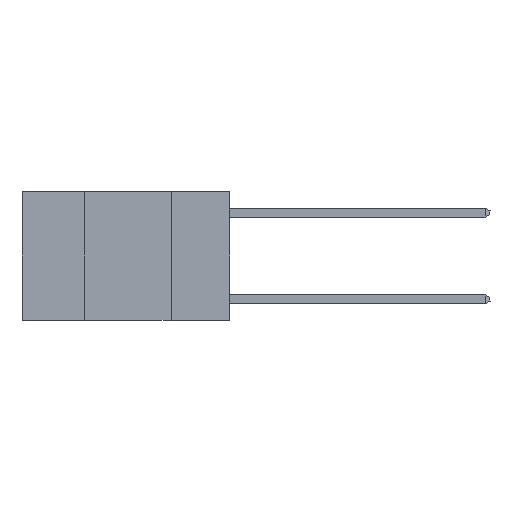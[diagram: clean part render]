
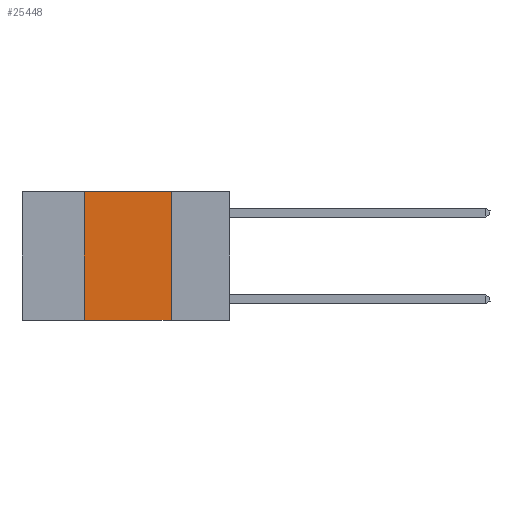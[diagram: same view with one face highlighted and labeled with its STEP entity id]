
A CAD part, left-side view. The second image highlights one B-rep face of the part: STEP entity #25448.
In plain terms, the highlighted planar face has unit normal (-1, 0, 0).
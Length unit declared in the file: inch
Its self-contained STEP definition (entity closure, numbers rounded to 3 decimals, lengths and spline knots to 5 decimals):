
#2127 = FACE_OUTER_BOUND ( 'NONE', #8134, .T. ) ;
#3153 = LINE ( 'NONE', #24647, #7280 ) ;
#5910 = EDGE_CURVE ( 'NONE', #15060, #19365, #3153, .T. ) ;
#6557 = VERTEX_POINT ( 'NONE', #20426 ) ;
#6738 = ORIENTED_EDGE ( 'NONE', *, *, #5910, .F. ) ;
#7203 = CARTESIAN_POINT ( 'NONE',  ( 0., 0.17, -0.37 ) ) ;
#7280 = VECTOR ( 'NONE', #15128, 39.37008 ) ;
#7332 = CARTESIAN_POINT ( 'NONE',  ( 0., 0.42, 0. ) ) ;
#8134 = EDGE_LOOP ( 'NONE', ( #16876, #6738, #12504, #13567 ) ) ;
#9075 = LINE ( 'NONE', #18094, #24394 ) ;
#9433 = EDGE_CURVE ( 'NONE', #6557, #15060, #9075, .T. ) ;
#12504 = ORIENTED_EDGE ( 'NONE', *, *, #9433, .F. ) ;
#13567 = ORIENTED_EDGE ( 'NONE', *, *, #25311, .T. ) ;
#13873 = CARTESIAN_POINT ( 'NONE',  ( 0., 0.6, -0.37 ) ) ;
#15060 = VERTEX_POINT ( 'NONE', #7332 ) ;
#15128 = DIRECTION ( 'NONE',  ( 0., -1., 0. ) ) ;
#15436 = CARTESIAN_POINT ( 'NONE',  ( 0., 0.6, 0. ) ) ;
#15563 = AXIS2_PLACEMENT_3D ( 'NONE', #15436, #29127, #24513 ) ;
#15665 = EDGE_CURVE ( 'NONE', #19365, #27081, #23588, .T. ) ;
#16086 = DIRECTION ( 'NONE',  ( 0., -1., 0. ) ) ;
#16234 = LINE ( 'NONE', #13873, #22209 ) ;
#16876 = ORIENTED_EDGE ( 'NONE', *, *, #15665, .F. ) ;
#18094 = CARTESIAN_POINT ( 'NONE',  ( 0., 0.42, 0. ) ) ;
#18815 = DIRECTION ( 'NONE',  ( 0., 0., -1. ) ) ;
#19365 = VERTEX_POINT ( 'NONE', #28139 ) ;
#20426 = CARTESIAN_POINT ( 'NONE',  ( 0., 0.42, -0.37 ) ) ;
#20608 = DIRECTION ( 'NONE',  ( 0., 0., 1. ) ) ;
#22209 = VECTOR ( 'NONE', #16086, 39.37008 ) ;
#23588 = LINE ( 'NONE', #25977, #27431 ) ;
#24394 = VECTOR ( 'NONE', #20608, 39.37008 ) ;
#24513 = DIRECTION ( 'NONE',  ( 0., 0., -1. ) ) ;
#24647 = CARTESIAN_POINT ( 'NONE',  ( 0., 0.6, 0. ) ) ;
#25311 = EDGE_CURVE ( 'NONE', #6557, #27081, #16234, .T. ) ;
#25448 = ADVANCED_FACE ( 'NONE', ( #2127 ), #27492, .F. ) ;
#25977 = CARTESIAN_POINT ( 'NONE',  ( 0., 0.17, 0. ) ) ;
#27081 = VERTEX_POINT ( 'NONE', #7203 ) ;
#27431 = VECTOR ( 'NONE', #18815, 39.37008 ) ;
#27492 = PLANE ( 'NONE',  #15563 ) ;
#28139 = CARTESIAN_POINT ( 'NONE',  ( 0., 0.17, 0. ) ) ;
#29127 = DIRECTION ( 'NONE',  ( 1., 0., 0. ) ) ;
